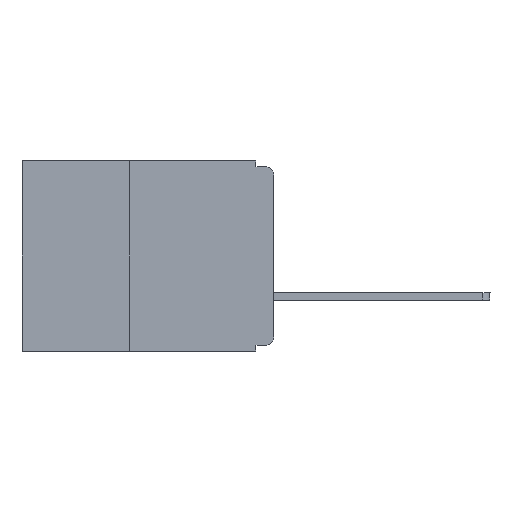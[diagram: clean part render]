
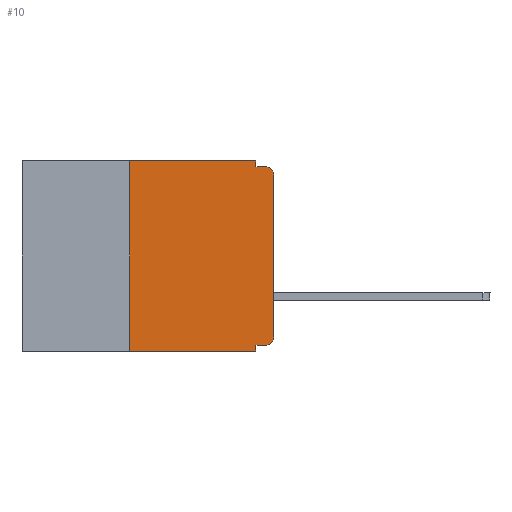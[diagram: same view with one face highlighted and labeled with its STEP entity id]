
A CAD part, left-side view. The second image highlights one B-rep face of the part: STEP entity #10.
In plain terms, the highlighted planar face has unit normal (-1, 0, 0).
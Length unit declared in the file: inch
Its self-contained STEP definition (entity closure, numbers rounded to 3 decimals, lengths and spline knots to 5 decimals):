
#10 = ADVANCED_FACE ( 'NONE', ( #10290 ), #4188, .F. ) ;
#12 = CARTESIAN_POINT ( 'NONE',  ( 0., 0.437, 0. ) ) ;
#140 = CARTESIAN_POINT ( 'NONE',  ( 0., 0., -0.32 ) ) ;
#503 = AXIS2_PLACEMENT_3D ( 'NONE', #12, #9347, #12419 ) ;
#855 = ORIENTED_EDGE ( 'NONE', *, *, #5815, .F. ) ;
#918 = EDGE_CURVE ( 'NONE', #5904, #1784, #12179, .T. ) ;
#1253 = VECTOR ( 'NONE', #5822, 39.37008 ) ;
#1265 = DIRECTION ( 'NONE',  ( 0., 1., 0. ) ) ;
#1502 = DIRECTION ( 'NONE',  ( 0., 0., 1. ) ) ;
#1560 = ORIENTED_EDGE ( 'NONE', *, *, #3989, .F. ) ;
#1784 = VERTEX_POINT ( 'NONE', #2361 ) ;
#1965 = CARTESIAN_POINT ( 'NONE',  ( 0., 0.031, 0. ) ) ;
#2111 = EDGE_CURVE ( 'NONE', #13289, #10052, #12140, .T. ) ;
#2361 = CARTESIAN_POINT ( 'NONE',  ( 0., 0.031, -0.01 ) ) ;
#2428 = ORIENTED_EDGE ( 'NONE', *, *, #918, .F. ) ;
#2437 = DIRECTION ( 'NONE',  ( 0., -1., 0. ) ) ;
#2588 = LINE ( 'NONE', #140, #10454 ) ;
#2654 = VERTEX_POINT ( 'NONE', #4375 ) ;
#2665 = EDGE_CURVE ( 'NONE', #8316, #5904, #4398, .T. ) ;
#2713 = ORIENTED_EDGE ( 'NONE', *, *, #12362, .F. ) ;
#2730 = DIRECTION ( 'NONE',  ( 0., 0., -1. ) ) ;
#3005 = ORIENTED_EDGE ( 'NONE', *, *, #9595, .T. ) ;
#3120 = ORIENTED_EDGE ( 'NONE', *, *, #2111, .T. ) ;
#3639 = CARTESIAN_POINT ( 'NONE',  ( 0., 0.437, 0. ) ) ;
#3787 = LINE ( 'NONE', #6764, #9585 ) ;
#3824 = VERTEX_POINT ( 'NONE', #11026 ) ;
#3919 = EDGE_LOOP ( 'NONE', ( #12317, #4637, #1560, #2428, #9248, #2713, #3120, #855, #12673, #3005 ) ) ;
#3989 = EDGE_CURVE ( 'NONE', #1784, #7734, #4322, .T. ) ;
#4080 = EDGE_CURVE ( 'NONE', #12399, #2654, #2588, .T. ) ;
#4188 = PLANE ( 'NONE',  #503 ) ;
#4212 = DIRECTION ( 'NONE',  ( 0., 0., -1. ) ) ;
#4254 = VERTEX_POINT ( 'NONE', #12976 ) ;
#4253 = CARTESIAN_POINT ( 'NONE',  ( 0., 0.031, -0.33 ) ) ;
#4322 = LINE ( 'NONE', #11372, #10920 ) ;
#4375 = CARTESIAN_POINT ( 'NONE',  ( 0., 0.031, -0.32 ) ) ;
#4398 = LINE ( 'NONE', #3639, #5972 ) ;
#4453 = CARTESIAN_POINT ( 'NONE',  ( 0., 0., 0. ) ) ;
#4637 = ORIENTED_EDGE ( 'NONE', *, *, #9907, .T. ) ;
#4844 = DIRECTION ( 'NONE',  ( -1., 0., 0. ) ) ;
#5197 = AXIS2_PLACEMENT_3D ( 'NONE', #7237, #12439, #4212 ) ;
#5251 = VECTOR ( 'NONE', #7579, 39.37008 ) ;
#5511 = VECTOR ( 'NONE', #2437, 39.37008 ) ;
#5748 = DIRECTION ( 'NONE',  ( 0., -1., 0. ) ) ;
#5764 = CIRCLE ( 'NONE', #5197, 0.015 ) ;
#5815 = EDGE_CURVE ( 'NONE', #2654, #10052, #3787, .T. ) ;
#5822 = DIRECTION ( 'NONE',  ( 0., 0., -1. ) ) ;
#5904 = VERTEX_POINT ( 'NONE', #1965 ) ;
#5949 = VECTOR ( 'NONE', #1502, 39.37008 ) ;
#5972 = VECTOR ( 'NONE', #5748, 39.37008 ) ;
#6592 = CARTESIAN_POINT ( 'NONE',  ( 0., 0.031, 0. ) ) ;
#6650 = AXIS2_PLACEMENT_3D ( 'NONE', #11033, #4844, #8773 ) ;
#6764 = CARTESIAN_POINT ( 'NONE',  ( 0., 0.031, -0.33 ) ) ;
#7237 = CARTESIAN_POINT ( 'NONE',  ( 0., 0.015, -0.025 ) ) ;
#7336 = DIRECTION ( 'NONE',  ( 0., -1., 0. ) ) ;
#7579 = DIRECTION ( 'NONE',  ( 0., 0., 1. ) ) ;
#7636 = EDGE_CURVE ( 'NONE', #3824, #4254, #8873, .T. ) ;
#7662 = CARTESIAN_POINT ( 'NONE',  ( 0., 0.25, -0.33 ) ) ;
#7734 = VERTEX_POINT ( 'NONE', #12649 ) ;
#8316 = VERTEX_POINT ( 'NONE', #10703 ) ;
#8653 = CARTESIAN_POINT ( 'NONE',  ( 0., 0.437, -0.33 ) ) ;
#8657 = LINE ( 'NONE', #7662, #5251 ) ;
#8773 = DIRECTION ( 'NONE',  ( 0., 0., -1. ) ) ;
#8873 = LINE ( 'NONE', #4453, #5949 ) ;
#9248 = ORIENTED_EDGE ( 'NONE', *, *, #2665, .F. ) ;
#9347 = DIRECTION ( 'NONE',  ( 1., 0., 0. ) ) ;
#9585 = VECTOR ( 'NONE', #2730, 39.37008 ) ;
#9595 = EDGE_CURVE ( 'NONE', #12399, #3824, #12719, .T. ) ;
#9907 = EDGE_CURVE ( 'NONE', #4254, #7734, #5764, .T. ) ;
#10052 = VERTEX_POINT ( 'NONE', #4253 ) ;
#10290 = FACE_OUTER_BOUND ( 'NONE', #3919, .T. ) ;
#10454 = VECTOR ( 'NONE', #1265, 39.37008 ) ;
#10703 = CARTESIAN_POINT ( 'NONE',  ( 0., 0.25, 0. ) ) ;
#10920 = VECTOR ( 'NONE', #7336, 39.37008 ) ;
#11026 = CARTESIAN_POINT ( 'NONE',  ( 0., 0., -0.305 ) ) ;
#11033 = CARTESIAN_POINT ( 'NONE',  ( 0., 0.015, -0.305 ) ) ;
#11372 = CARTESIAN_POINT ( 'NONE',  ( 0., 0., -0.01 ) ) ;
#11879 = CARTESIAN_POINT ( 'NONE',  ( 0., 0.015, -0.32 ) ) ;
#12140 = LINE ( 'NONE', #8653, #5511 ) ;
#12179 = LINE ( 'NONE', #6592, #1253 ) ;
#12317 = ORIENTED_EDGE ( 'NONE', *, *, #7636, .T. ) ;
#12362 = EDGE_CURVE ( 'NONE', #13289, #8316, #8657, .T. ) ;
#12399 = VERTEX_POINT ( 'NONE', #11879 ) ;
#12419 = DIRECTION ( 'NONE',  ( 0., 0., -1. ) ) ;
#12439 = DIRECTION ( 'NONE',  ( -1., 0., 0. ) ) ;
#12649 = CARTESIAN_POINT ( 'NONE',  ( 0., 0.015, -0.01 ) ) ;
#12673 = ORIENTED_EDGE ( 'NONE', *, *, #4080, .F. ) ;
#12719 = CIRCLE ( 'NONE', #6650, 0.015 ) ;
#12947 = CARTESIAN_POINT ( 'NONE',  ( 0., 0.25, -0.33 ) ) ;
#12976 = CARTESIAN_POINT ( 'NONE',  ( 0., 0., -0.025 ) ) ;
#13289 = VERTEX_POINT ( 'NONE', #12947 ) ;
